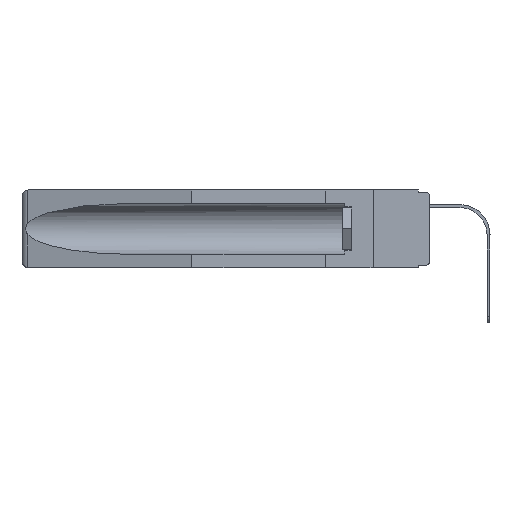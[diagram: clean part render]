
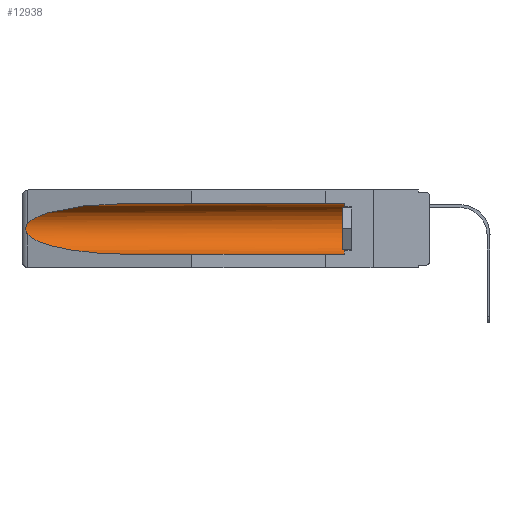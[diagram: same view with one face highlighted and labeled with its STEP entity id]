
A CAD part, left-side view. The second image highlights one B-rep face of the part: STEP entity #12938.
In plain terms, the highlighted cylindrical face has radius 2.857 mm (diameter 5.715 mm), a partial arc.
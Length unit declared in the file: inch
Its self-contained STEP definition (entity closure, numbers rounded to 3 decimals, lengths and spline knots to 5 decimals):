
#1196 = DIRECTION ( 'NONE',  ( 0., 0., 1. ) ) ;
#1268 = DIRECTION ( 'NONE',  ( 0., 1., 0. ) ) ;
#1364 = VERTEX_POINT ( 'NONE', #15990 ) ;
#1394 = CARTESIAN_POINT ( 'NONE',  ( 0.2675, 1.53308, -0.16763 ) ) ;
#1754 = LINE ( 'NONE', #8437, #8114 ) ;
#1869 = ORIENTED_EDGE ( 'NONE', *, *, #11599, .F. ) ;
#1888 = CARTESIAN_POINT ( 'NONE',  ( 0.21114, 1.30732, -0.284 ) ) ;
#2350 = EDGE_LOOP ( 'NONE', ( #21667, #17243, #4427, #1869, #10557, #10316 ) ) ;
#2419 = B_SPLINE_CURVE_WITH_KNOTS ( 'NONE', 3,
 ( #12921, #9945, #19594, #9739, #1394, #14974, #16416, #4580, #11705, #21571 ),
 .UNSPECIFIED., .F., .F.,
 ( 4, 2, 2, 2, 4 ),
 ( 0., 0.00029, 0.00058, 0.00087, 0.00117 ),
 .UNSPECIFIED. ) ;
#2612 = AXIS2_PLACEMENT_3D ( 'NONE', #4376, #11191, #1196 ) ;
#3004 = VERTEX_POINT ( 'NONE', #16047 ) ;
#4349 = VERTEX_POINT ( 'NONE', #15478 ) ;
#4376 = CARTESIAN_POINT ( 'NONE',  ( 0.155, 0.126, -0.1715 ) ) ;
#4427 = ORIENTED_EDGE ( 'NONE', *, *, #20876, .T. ) ;
#4580 = CARTESIAN_POINT ( 'NONE',  ( 0.26655, 1.53094, -0.18657 ) ) ;
#4660 = CARTESIAN_POINT ( 'NONE',  ( 0.155, 1.07973, -0.059 ) ) ;
#4851 = CARTESIAN_POINT ( 'NONE',  ( 0.25451, 1.48313, -0.24835 ) ) ;
#5954 = LINE ( 'NONE', #12779, #7809 ) ;
#6812 = CARTESIAN_POINT ( 'NONE',  ( 0.26537, 1.52718, -0.19328 ) ) ;
#7809 = VECTOR ( 'NONE', #1268, 39.37008 ) ;
#7879 = CYLINDRICAL_SURFACE ( 'NONE', #16562, 0.1125 ) ;
#8114 = VECTOR ( 'NONE', #15111, 39.37008 ) ;
#8437 = CARTESIAN_POINT ( 'NONE',  ( 0.155, -0.30754, -0.284 ) ) ;
#8565 = CARTESIAN_POINT ( 'NONE',  ( 0.155, 1.07973, -0.284 ) ) ;
#9598 = VERTEX_POINT ( 'NONE', #21177 ) ;
#9739 = CARTESIAN_POINT ( 'NONE',  ( 0.2673, 1.5327, -0.16383 ) ) ;
#9945 = CARTESIAN_POINT ( 'NONE',  ( 0.26597, 1.52961, -0.15275 ) ) ;
#10316 = ORIENTED_EDGE ( 'NONE', *, *, #14576, .T. ) ;
#10516 = VERTEX_POINT ( 'NONE', #16012 ) ;
#10557 = ORIENTED_EDGE ( 'NONE', *, *, #17649, .T. ) ;
#11190 = DIRECTION ( 'NONE',  ( 0., 0., 1. ) ) ;
#11191 = DIRECTION ( 'NONE',  ( 0., -1., 0. ) ) ;
#11578 = CARTESIAN_POINT ( 'NONE',  ( 0.26537, 1.52718, -0.14972 ) ) ;
#11599 = EDGE_CURVE ( 'NONE', #16196, #4349, #1754, .T. ) ;
#11677 = CARTESIAN_POINT ( 'NONE',  ( 0.21114, 1.30732, -0.059 ) ) ;
#11705 = CARTESIAN_POINT ( 'NONE',  ( 0.26597, 1.5296, -0.19026 ) ) ;
#12190 =( BOUNDED_CURVE ( )  B_SPLINE_CURVE ( 3, ( #6812, #4851, #1888, #8565 ),
 .UNSPECIFIED., .F., .F. ) 
 B_SPLINE_CURVE_WITH_KNOTS ( ( 4, 4 ),
 ( 0.1948, 1.5708 ),
 .UNSPECIFIED. ) 
 CURVE ( )  GEOMETRIC_REPRESENTATION_ITEM ( )  RATIONAL_B_SPLINE_CURVE ( ( 1., 0.848, 0.848, 1. ) ) 
 REPRESENTATION_ITEM ( '' )  );
#12779 = CARTESIAN_POINT ( 'NONE',  ( 0.155, -0.30754, -0.059 ) ) ;
#12921 = CARTESIAN_POINT ( 'NONE',  ( 0.26537, 1.52718, -0.14972 ) ) ;
#12928 = CARTESIAN_POINT ( 'NONE',  ( 0.155, -0.30754, -0.1715 ) ) ;
#12938 = ADVANCED_FACE ( 'NONE', ( #16326 ), #7879, .F. ) ;
#14576 = EDGE_CURVE ( 'NONE', #3004, #1364, #5954, .T. ) ;
#14641 = EDGE_CURVE ( 'NONE', #1364, #10516, #17371, .T. ) ;
#14974 = CARTESIAN_POINT ( 'NONE',  ( 0.2675, 1.53308, -0.17534 ) ) ;
#15054 = DIRECTION ( 'NONE',  ( 0., 1., 0. ) ) ;
#15111 = DIRECTION ( 'NONE',  ( 0., 1., 0. ) ) ;
#15265 = CARTESIAN_POINT ( 'NONE',  ( 0.25451, 1.48313, -0.09465 ) ) ;
#15478 = CARTESIAN_POINT ( 'NONE',  ( 0.155, 1.07973, -0.284 ) ) ;
#15790 = EDGE_CURVE ( 'NONE', #10516, #9598, #2419, .T. ) ;
#15990 = CARTESIAN_POINT ( 'NONE',  ( 0.155, 1.07973, -0.059 ) ) ;
#16012 = CARTESIAN_POINT ( 'NONE',  ( 0.26537, 1.52718, -0.14972 ) ) ;
#16047 = CARTESIAN_POINT ( 'NONE',  ( 0.155, 0.126, -0.059 ) ) ;
#16196 = VERTEX_POINT ( 'NONE', #20505 ) ;
#16326 = FACE_OUTER_BOUND ( 'NONE', #2350, .T. ) ;
#16416 = CARTESIAN_POINT ( 'NONE',  ( 0.2673, 1.53269, -0.17917 ) ) ;
#16562 = AXIS2_PLACEMENT_3D ( 'NONE', #12928, #15054, #11190 ) ;
#17243 = ORIENTED_EDGE ( 'NONE', *, *, #15790, .T. ) ;
#17371 =( BOUNDED_CURVE ( )  B_SPLINE_CURVE ( 3, ( #4660, #11677, #15265, #11578 ),
 .UNSPECIFIED., .F., .F. ) 
 B_SPLINE_CURVE_WITH_KNOTS ( ( 4, 4 ),
 ( 4.71239, 6.08839 ),
 .UNSPECIFIED. ) 
 CURVE ( )  GEOMETRIC_REPRESENTATION_ITEM ( )  RATIONAL_B_SPLINE_CURVE ( ( 1., 0.848, 0.848, 1. ) ) 
 REPRESENTATION_ITEM ( '' )  );
#17649 = EDGE_CURVE ( 'NONE', #16196, #3004, #18697, .T. ) ;
#18697 = CIRCLE ( 'NONE', #2612, 0.1125 ) ;
#19594 = CARTESIAN_POINT ( 'NONE',  ( 0.26654, 1.53092, -0.15636 ) ) ;
#20505 = CARTESIAN_POINT ( 'NONE',  ( 0.155, 0.126, -0.284 ) ) ;
#20876 = EDGE_CURVE ( 'NONE', #9598, #4349, #12190, .T. ) ;
#21177 = CARTESIAN_POINT ( 'NONE',  ( 0.26537, 1.52718, -0.19328 ) ) ;
#21571 = CARTESIAN_POINT ( 'NONE',  ( 0.26537, 1.52718, -0.19328 ) ) ;
#21667 = ORIENTED_EDGE ( 'NONE', *, *, #14641, .T. ) ;
